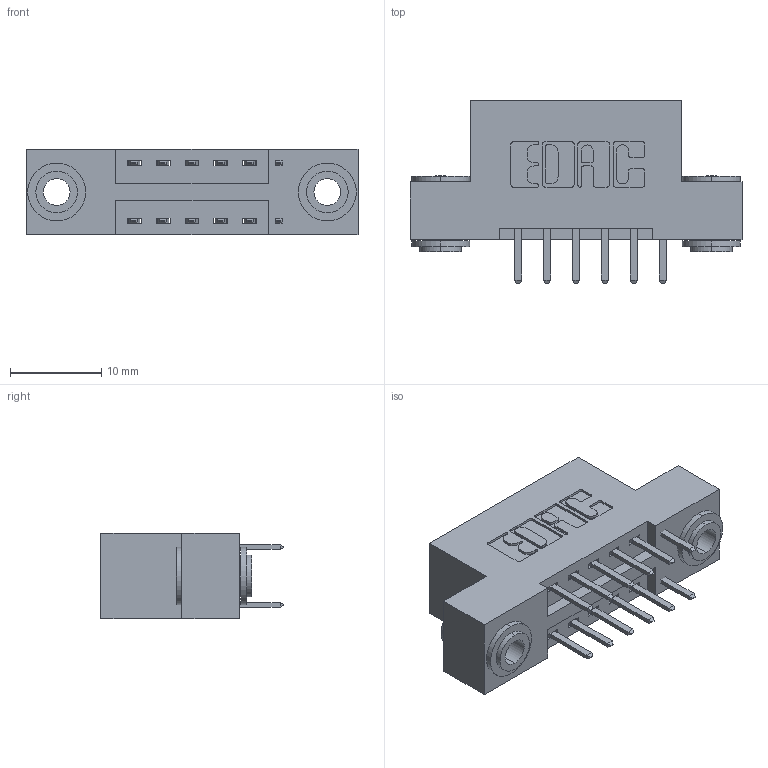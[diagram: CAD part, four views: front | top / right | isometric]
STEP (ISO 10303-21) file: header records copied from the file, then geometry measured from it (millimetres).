
FILE_DESCRIPTION (( 'STEP AP203' ), '1' );
FILE_NAME ('346-012-520-203.STEP', '2022-05-17T19:01:00', ( '' ), ( '' ), 'SwSTEP 2.0', 'SolidWorks 2020', '' );
FILE_SCHEMA (( 'CONFIG_CONTROL_DESIGN' ));
Length unit declared in the file: inch
Products named in the file (4): 345-250-002_345-250-002-102; 346-012-520-203; 345-292-001_345-293-120; 346 Part_Flush Mounting Lugs - 0.156 Dia-TH
Assembly tree (15 placements, depth 2):
  346-012-520-203
    346 Part_Flush Mounting Lugs - 0.156 Dia-TH
    345-292-001_345-293-120  x12
    345-250-002_345-250-002-102  x2
Bounding box: 36.45 x 20.02 x 9.4 mm (x, y, z)
Volume: 3280.9 mm3; surface area: 4268.4 mm2
Topology: 15 solids, 15 shells, 834 faces, 2355 edges, 1534 vertices
Faces by surface type: plane 534, cylinder 292, cone 8
Entity records: 9488 total; most frequent: CARTESIAN_POINT 1599, ORIENTED_EDGE 1510, DIRECTION 1481, EDGE_CURVE 755, LINE 575, VECTOR 575, VERTEX_POINT 498, AXIS2_PLACEMENT_3D 453
